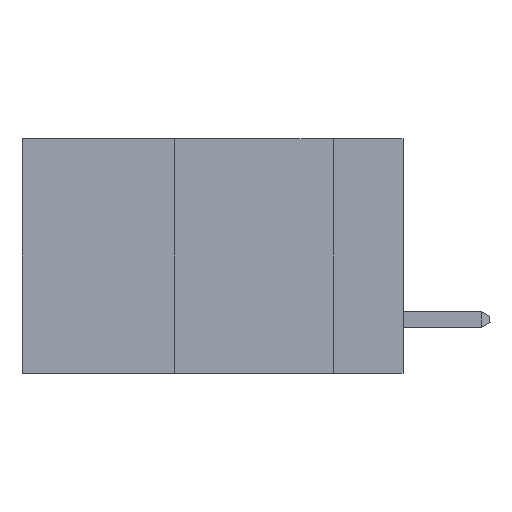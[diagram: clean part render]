
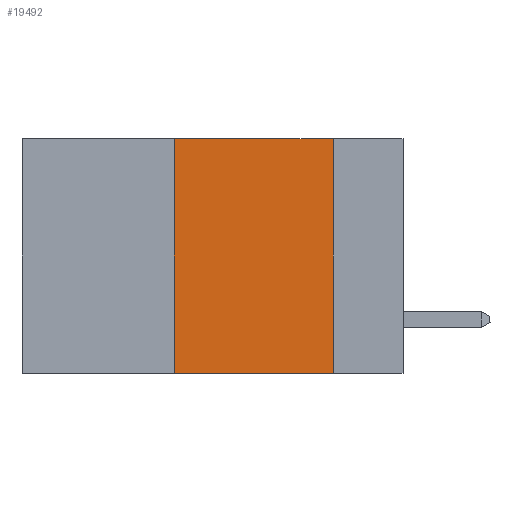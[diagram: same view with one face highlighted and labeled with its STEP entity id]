
A CAD part, left-side view. The second image highlights one B-rep face of the part: STEP entity #19492.
In plain terms, the highlighted planar face has unit normal (-1, 0, 0).
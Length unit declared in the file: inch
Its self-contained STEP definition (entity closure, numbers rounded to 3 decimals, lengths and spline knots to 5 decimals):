
#123 = LINE ( 'NONE', #42378, #48167 ) ;
#4950 = CARTESIAN_POINT ( 'NONE',  ( 0., 0.36, -0.37 ) ) ;
#6034 = DIRECTION ( 'NONE',  ( 1., 0., 0. ) ) ;
#6352 = PLANE ( 'NONE',  #48103 ) ;
#7723 = ORIENTED_EDGE ( 'NONE', *, *, #22416, .F. ) ;
#7758 = DIRECTION ( 'NONE',  ( 0., -1., 0. ) ) ;
#8682 = VERTEX_POINT ( 'NONE', #28005 ) ;
#10250 = LINE ( 'NONE', #34950, #16287 ) ;
#13400 = FACE_OUTER_BOUND ( 'NONE', #40647, .T. ) ;
#13436 = VECTOR ( 'NONE', #7758, 39.37008 ) ;
#13445 = CARTESIAN_POINT ( 'NONE',  ( 0., 0.11, 0. ) ) ;
#13454 = ORIENTED_EDGE ( 'NONE', *, *, #19698, .T. ) ;
#15570 = VECTOR ( 'NONE', #47967, 39.37008 ) ;
#16287 = VECTOR ( 'NONE', #19905, 39.37008 ) ;
#17475 = CARTESIAN_POINT ( 'NONE',  ( 0., 0.6, 0. ) ) ;
#19492 = ADVANCED_FACE ( 'NONE', ( #13400 ), #6352, .F. ) ;
#19698 = EDGE_CURVE ( 'NONE', #43246, #26372, #123, .T. ) ;
#19905 = DIRECTION ( 'NONE',  ( 0., 0., 1. ) ) ;
#20019 = LINE ( 'NONE', #37466, #13436 ) ;
#22416 = EDGE_CURVE ( 'NONE', #8682, #26372, #25758, .T. ) ;
#25758 = LINE ( 'NONE', #13445, #15570 ) ;
#26372 = VERTEX_POINT ( 'NONE', #27680 ) ;
#27680 = CARTESIAN_POINT ( 'NONE',  ( 0., 0.11, -0.37 ) ) ;
#28005 = CARTESIAN_POINT ( 'NONE',  ( 0., 0.11, 0. ) ) ;
#28856 = EDGE_CURVE ( 'NONE', #38683, #8682, #20019, .T. ) ;
#28994 = ORIENTED_EDGE ( 'NONE', *, *, #37445, .F. ) ;
#34950 = CARTESIAN_POINT ( 'NONE',  ( 0., 0.36, 0. ) ) ;
#36709 = DIRECTION ( 'NONE',  ( 0., 0., -1. ) ) ;
#37445 = EDGE_CURVE ( 'NONE', #43246, #38683, #10250, .T. ) ;
#37466 = CARTESIAN_POINT ( 'NONE',  ( 0., 0.6, 0. ) ) ;
#38683 = VERTEX_POINT ( 'NONE', #49581 ) ;
#40647 = EDGE_LOOP ( 'NONE', ( #7723, #44891, #28994, #13454 ) ) ;
#42035 = DIRECTION ( 'NONE',  ( 0., -1., 0. ) ) ;
#42378 = CARTESIAN_POINT ( 'NONE',  ( 0., 0.6, -0.37 ) ) ;
#43246 = VERTEX_POINT ( 'NONE', #4950 ) ;
#44891 = ORIENTED_EDGE ( 'NONE', *, *, #28856, .F. ) ;
#47967 = DIRECTION ( 'NONE',  ( 0., 0., -1. ) ) ;
#48103 = AXIS2_PLACEMENT_3D ( 'NONE', #17475, #6034, #36709 ) ;
#48167 = VECTOR ( 'NONE', #42035, 39.37008 ) ;
#49581 = CARTESIAN_POINT ( 'NONE',  ( 0., 0.36, 0. ) ) ;
